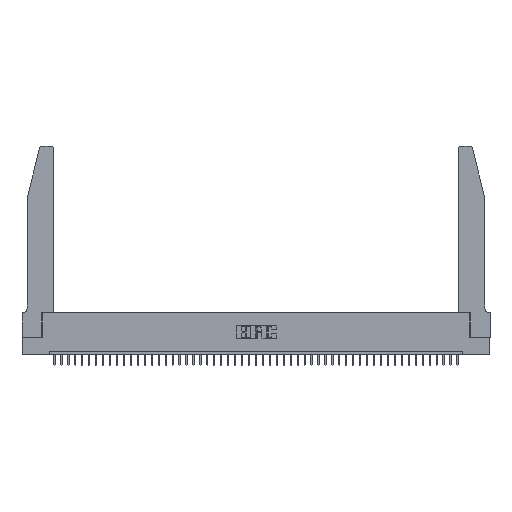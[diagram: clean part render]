
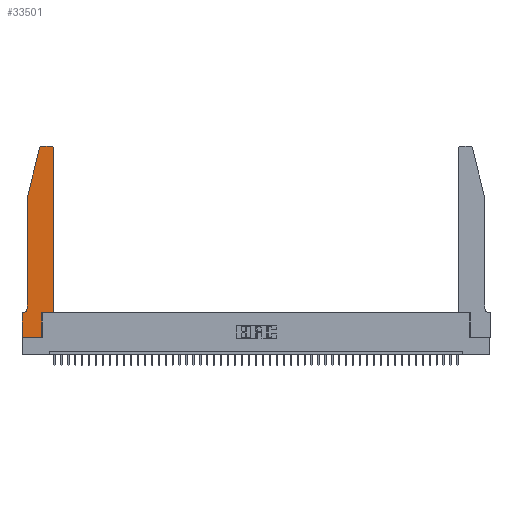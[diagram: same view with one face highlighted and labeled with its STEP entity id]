
A CAD part, top view. The second image highlights one B-rep face of the part: STEP entity #33501.
In plain terms, the highlighted planar face has unit normal (0, 0, 1).
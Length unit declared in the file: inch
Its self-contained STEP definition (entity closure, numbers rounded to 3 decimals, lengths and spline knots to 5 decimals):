
#875 = ORIENTED_EDGE ( 'NONE', *, *, #4505, .T. ) ;
#1881 = AXIS2_PLACEMENT_3D ( 'NONE', #28019, #17701, #21017 ) ;
#2248 = CIRCLE ( 'NONE', #1881, 0.03 ) ;
#2289 = DIRECTION ( 'NONE',  ( 0., -1., 0. ) ) ;
#2476 = CARTESIAN_POINT ( 'NONE',  ( 0.4505, 2.72, 0.37 ) ) ;
#3449 = LINE ( 'NONE', #5524, #45414 ) ;
#4044 = ORIENTED_EDGE ( 'NONE', *, *, #37780, .T. ) ;
#4505 = EDGE_CURVE ( 'NONE', #40583, #43724, #36648, .T. ) ;
#4526 = VECTOR ( 'NONE', #8955, 39.37008 ) ;
#4681 = CARTESIAN_POINT ( 'NONE',  ( 0.4505, 0.35, 0.37 ) ) ;
#4744 = EDGE_CURVE ( 'NONE', #23210, #24906, #30377, .T. ) ;
#5524 = CARTESIAN_POINT ( 'NONE',  ( 0.2605, 2.75, 0.37 ) ) ;
#5682 = ORIENTED_EDGE ( 'NONE', *, *, #36654, .T. ) ;
#6329 = CARTESIAN_POINT ( 'NONE',  ( 0.0755, 0.42, 0.37 ) ) ;
#6519 = FACE_OUTER_BOUND ( 'NONE', #21372, .T. ) ;
#7905 = VECTOR ( 'NONE', #37686, 39.37008 ) ;
#7968 = EDGE_CURVE ( 'NONE', #43102, #40583, #3449, .T. ) ;
#8234 = EDGE_CURVE ( 'NONE', #41526, #46726, #41561, .T. ) ;
#8549 = VECTOR ( 'NONE', #15461, 39.37008 ) ;
#8955 = DIRECTION ( 'NONE',  ( 0., 1., 0. ) ) ;
#8986 = CARTESIAN_POINT ( 'NONE',  ( 0.4505, 0.35, 0.37 ) ) ;
#9537 = CARTESIAN_POINT ( 'NONE',  ( 0.284, 2.75, 0.37 ) ) ;
#11890 = AXIS2_PLACEMENT_3D ( 'NONE', #28746, #27250, #17816 ) ;
#11955 = VERTEX_POINT ( 'NONE', #2476 ) ;
#12464 = VECTOR ( 'NONE', #42443, 39.37008 ) ;
#12729 = EDGE_CURVE ( 'NONE', #27510, #42404, #17499, .T. ) ;
#14108 = CARTESIAN_POINT ( 'NONE',  ( 0.2865, 0., 0.37 ) ) ;
#14398 = CARTESIAN_POINT ( 'NONE',  ( 0.25487, 2.72718, 0.37 ) ) ;
#15461 = DIRECTION ( 'NONE',  ( -0.239, -0.971, 0. ) ) ;
#15954 = EDGE_CURVE ( 'NONE', #33247, #23210, #28278, .T. ) ;
#16089 = CARTESIAN_POINT ( 'NONE',  ( 0., 0., 0.37 ) ) ;
#16955 = DIRECTION ( 'NONE',  ( 0., 0., 1. ) ) ;
#17499 = LINE ( 'NONE', #34103, #4526 ) ;
#17701 = DIRECTION ( 'NONE',  ( 0., 0., 1. ) ) ;
#17777 = EDGE_CURVE ( 'NONE', #42404, #36883, #20700, .T. ) ;
#17816 = DIRECTION ( 'NONE',  ( -1., 0., 0. ) ) ;
#18122 = CARTESIAN_POINT ( 'NONE',  ( 0.4505, 0.35, 0.37 ) ) ;
#20602 = EDGE_CURVE ( 'NONE', #43724, #41526, #45428, .T. ) ;
#20700 = LINE ( 'NONE', #8986, #26957 ) ;
#21017 = DIRECTION ( 'NONE',  ( 1., 0., 0. ) ) ;
#21372 = EDGE_LOOP ( 'NONE', ( #43490, #875, #22058, #23567, #5682, #23481, #29836, #22478, #21888, #38796, #4044, #41151 ) ) ;
#21888 = ORIENTED_EDGE ( 'NONE', *, *, #12729, .T. ) ;
#22058 = ORIENTED_EDGE ( 'NONE', *, *, #20602, .T. ) ;
#22287 = CARTESIAN_POINT ( 'NONE',  ( 0., 0., 0.37 ) ) ;
#22478 = ORIENTED_EDGE ( 'NONE', *, *, #34658, .T. ) ;
#22865 = CARTESIAN_POINT ( 'NONE',  ( 0.0755, 2., 0.37 ) ) ;
#22971 = EDGE_CURVE ( 'NONE', #11955, #43102, #2248, .T. ) ;
#23210 = VERTEX_POINT ( 'NONE', #29870 ) ;
#23361 = DIRECTION ( 'NONE',  ( 1., 0., 0. ) ) ;
#23481 = ORIENTED_EDGE ( 'NONE', *, *, #15954, .T. ) ;
#23567 = ORIENTED_EDGE ( 'NONE', *, *, #8234, .T. ) ;
#23622 = CARTESIAN_POINT ( 'NONE',  ( 0.2865, 0.35, 0.37 ) ) ;
#24906 = VERTEX_POINT ( 'NONE', #22287 ) ;
#25327 = DIRECTION ( 'NONE',  ( 1., 0., 0. ) ) ;
#26551 = CARTESIAN_POINT ( 'NONE',  ( 0.0755, 2., 0.37 ) ) ;
#26957 = VECTOR ( 'NONE', #23361, 39.37008 ) ;
#27250 = DIRECTION ( 'NONE',  ( 0., 0., -1. ) ) ;
#27253 = DIRECTION ( 'NONE',  ( 1., 0., 0. ) ) ;
#27510 = VERTEX_POINT ( 'NONE', #14108 ) ;
#28019 = CARTESIAN_POINT ( 'NONE',  ( 0.4205, 2.72, 0.37 ) ) ;
#28278 = LINE ( 'NONE', #40310, #7905 ) ;
#28746 = CARTESIAN_POINT ( 'NONE',  ( 0.0055, 0.42, 0.37 ) ) ;
#29004 = VECTOR ( 'NONE', #41695, 39.37008 ) ;
#29836 = ORIENTED_EDGE ( 'NONE', *, *, #4744, .T. ) ;
#29870 = CARTESIAN_POINT ( 'NONE',  ( 0., 0.35, 0.37 ) ) ;
#30377 = LINE ( 'NONE', #38207, #33777 ) ;
#33247 = VERTEX_POINT ( 'NONE', #40755 ) ;
#33501 = ADVANCED_FACE ( 'NONE', ( #6519 ), #45677, .T. ) ;
#33777 = VECTOR ( 'NONE', #2289, 39.37008 ) ;
#34103 = CARTESIAN_POINT ( 'NONE',  ( 0.2865, 0.35, 0.37 ) ) ;
#34658 = EDGE_CURVE ( 'NONE', #24906, #27510, #44197, .T. ) ;
#34912 = CIRCLE ( 'NONE', #11890, 0.07 ) ;
#35059 = DIRECTION ( 'NONE',  ( -1., 0., 0. ) ) ;
#35115 = AXIS2_PLACEMENT_3D ( 'NONE', #38368, #16955, #27253 ) ;
#35178 = CARTESIAN_POINT ( 'NONE',  ( 0.284, 2.72, 0.37 ) ) ;
#35623 = AXIS2_PLACEMENT_3D ( 'NONE', #35178, #43426, #25327 ) ;
#35704 = CARTESIAN_POINT ( 'NONE',  ( 0.4205, 2.75, 0.37 ) ) ;
#36648 = CIRCLE ( 'NONE', #35623, 0.03 ) ;
#36654 = EDGE_CURVE ( 'NONE', #46726, #33247, #34912, .T. ) ;
#36883 = VERTEX_POINT ( 'NONE', #18122 ) ;
#37686 = DIRECTION ( 'NONE',  ( -1., 0., 0. ) ) ;
#37780 = EDGE_CURVE ( 'NONE', #36883, #11955, #41109, .T. ) ;
#38207 = CARTESIAN_POINT ( 'NONE',  ( 0., 0., 0.37 ) ) ;
#38289 = VECTOR ( 'NONE', #44418, 39.37008 ) ;
#38368 = CARTESIAN_POINT ( 'NONE',  ( 0., 0.35, 0.37 ) ) ;
#38796 = ORIENTED_EDGE ( 'NONE', *, *, #17777, .T. ) ;
#40310 = CARTESIAN_POINT ( 'NONE',  ( 0.0755, 0.35, 0.37 ) ) ;
#40583 = VERTEX_POINT ( 'NONE', #9537 ) ;
#40755 = CARTESIAN_POINT ( 'NONE',  ( 0.0055, 0.35, 0.37 ) ) ;
#41109 = LINE ( 'NONE', #4681, #38289 ) ;
#41151 = ORIENTED_EDGE ( 'NONE', *, *, #22971, .T. ) ;
#41526 = VERTEX_POINT ( 'NONE', #22865 ) ;
#41561 = LINE ( 'NONE', #45343, #29004 ) ;
#41695 = DIRECTION ( 'NONE',  ( 0., -1., 0. ) ) ;
#42404 = VERTEX_POINT ( 'NONE', #23622 ) ;
#42443 = DIRECTION ( 'NONE',  ( 1., 0., 0. ) ) ;
#43102 = VERTEX_POINT ( 'NONE', #35704 ) ;
#43426 = DIRECTION ( 'NONE',  ( 0., 0., 1. ) ) ;
#43490 = ORIENTED_EDGE ( 'NONE', *, *, #7968, .T. ) ;
#43724 = VERTEX_POINT ( 'NONE', #14398 ) ;
#44197 = LINE ( 'NONE', #16089, #12464 ) ;
#44418 = DIRECTION ( 'NONE',  ( 0., 1., 0. ) ) ;
#45343 = CARTESIAN_POINT ( 'NONE',  ( 0.0755, 2., 0.37 ) ) ;
#45414 = VECTOR ( 'NONE', #35059, 39.37008 ) ;
#45428 = LINE ( 'NONE', #26551, #8549 ) ;
#45677 = PLANE ( 'NONE',  #35115 ) ;
#46726 = VERTEX_POINT ( 'NONE', #6329 ) ;
